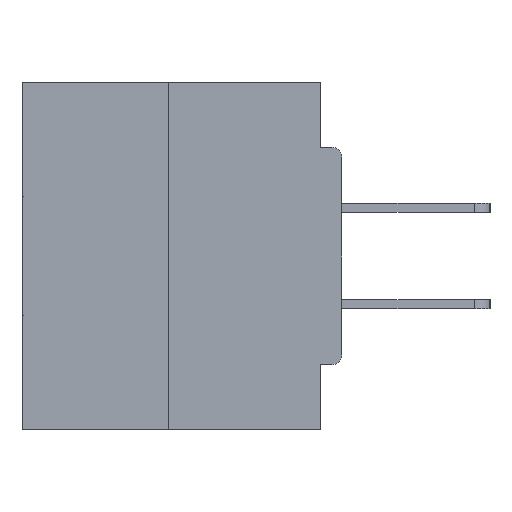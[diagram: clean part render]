
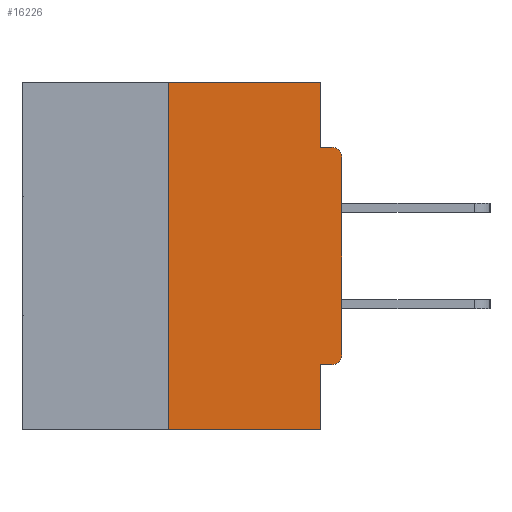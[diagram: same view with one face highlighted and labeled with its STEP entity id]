
A CAD part, left-side view. The second image highlights one B-rep face of the part: STEP entity #16226.
In plain terms, the highlighted planar face has unit normal (-1, 0, 0).
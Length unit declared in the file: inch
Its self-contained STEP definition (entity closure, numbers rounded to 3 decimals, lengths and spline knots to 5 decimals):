
#726 = CARTESIAN_POINT ( 'NONE',  ( 0., 0.015, -0.4065 ) ) ;
#1632 = CIRCLE ( 'NONE', #24550, 0.015 ) ;
#4187 = VERTEX_POINT ( 'NONE', #37827 ) ;
#4251 = EDGE_CURVE ( 'NONE', #29458, #31498, #21934, .T. ) ;
#4314 = EDGE_CURVE ( 'NONE', #35933, #25921, #5389, .T. ) ;
#4438 = LINE ( 'NONE', #27031, #31318 ) ;
#4513 = ORIENTED_EDGE ( 'NONE', *, *, #22392, .T. ) ;
#4729 = VERTEX_POINT ( 'NONE', #14237 ) ;
#4749 = DIRECTION ( 'NONE',  ( 0., 0., -1. ) ) ;
#5389 = LINE ( 'NONE', #38751, #9165 ) ;
#6288 = EDGE_CURVE ( 'NONE', #29458, #33371, #18903, .T. ) ;
#6418 = CARTESIAN_POINT ( 'NONE',  ( 0., 0., -0.3915 ) ) ;
#8263 = DIRECTION ( 'NONE',  ( 1., 0., 0. ) ) ;
#9165 = VECTOR ( 'NONE', #26657, 39.37008 ) ;
#9715 = VECTOR ( 'NONE', #4749, 39.37008 ) ;
#10452 = CARTESIAN_POINT ( 'NONE',  ( 0., 0.25, 0. ) ) ;
#10762 = FACE_OUTER_BOUND ( 'NONE', #16649, .T. ) ;
#10782 = CARTESIAN_POINT ( 'NONE',  ( 0., 0.015, -0.0935 ) ) ;
#11298 = DIRECTION ( 'NONE',  ( 0., -1., 0. ) ) ;
#11410 = CARTESIAN_POINT ( 'NONE',  ( 0., 0.015, -0.1085 ) ) ;
#11982 = DIRECTION ( 'NONE',  ( 0., -1., 0. ) ) ;
#13202 = VERTEX_POINT ( 'NONE', #36590 ) ;
#13882 = VECTOR ( 'NONE', #20357, 39.37008 ) ;
#14084 = LINE ( 'NONE', #37964, #38098 ) ;
#14098 = CARTESIAN_POINT ( 'NONE',  ( 0., 0.46, 0. ) ) ;
#14237 = CARTESIAN_POINT ( 'NONE',  ( 0., 0.031, -0.5 ) ) ;
#15349 = CARTESIAN_POINT ( 'NONE',  ( 0., 0.031, 0. ) ) ;
#16226 = ADVANCED_FACE ( 'NONE', ( #10762 ), #38574, .F. ) ;
#16649 = EDGE_LOOP ( 'NONE', ( #32845, #31484, #32725, #24927, #24960, #26338, #16756, #4513, #18245, #19762 ) ) ;
#16756 = ORIENTED_EDGE ( 'NONE', *, *, #21710, .T. ) ;
#16948 = CARTESIAN_POINT ( 'NONE',  ( 0., 0.25, 0. ) ) ;
#17215 = DIRECTION ( 'NONE',  ( 0., 0., -1. ) ) ;
#17398 = AXIS2_PLACEMENT_3D ( 'NONE', #31914, #35053, #37705 ) ;
#18002 = DIRECTION ( 'NONE',  ( 0., 0., 1. ) ) ;
#18245 = ORIENTED_EDGE ( 'NONE', *, *, #24643, .F. ) ;
#18903 = CIRCLE ( 'NONE', #17398, 0.015 ) ;
#19762 = ORIENTED_EDGE ( 'NONE', *, *, #34232, .F. ) ;
#20177 = DIRECTION ( 'NONE',  ( 0., 0., -1. ) ) ;
#20357 = DIRECTION ( 'NONE',  ( 0., 1., 0. ) ) ;
#20822 = CARTESIAN_POINT ( 'NONE',  ( 0., 0.031, -0.4065 ) ) ;
#21710 = EDGE_CURVE ( 'NONE', #33371, #13202, #27194, .T. ) ;
#21934 = LINE ( 'NONE', #26002, #13882 ) ;
#22392 = EDGE_CURVE ( 'NONE', #13202, #37519, #1632, .T. ) ;
#23120 = CARTESIAN_POINT ( 'NONE',  ( 0., 0.031, -0.5 ) ) ;
#23213 = LINE ( 'NONE', #26319, #30232 ) ;
#24550 = AXIS2_PLACEMENT_3D ( 'NONE', #11410, #35357, #17215 ) ;
#24643 = EDGE_CURVE ( 'NONE', #4187, #37519, #4438, .T. ) ;
#24927 = ORIENTED_EDGE ( 'NONE', *, *, #35275, .F. ) ;
#24960 = ORIENTED_EDGE ( 'NONE', *, *, #4251, .F. ) ;
#25842 = EDGE_CURVE ( 'NONE', #33291, #35933, #35011, .T. ) ;
#25921 = VERTEX_POINT ( 'NONE', #15349 ) ;
#26002 = CARTESIAN_POINT ( 'NONE',  ( 0., 0., -0.4065 ) ) ;
#26319 = CARTESIAN_POINT ( 'NONE',  ( 0., 0.46, -0.5 ) ) ;
#26338 = ORIENTED_EDGE ( 'NONE', *, *, #6288, .T. ) ;
#26657 = DIRECTION ( 'NONE',  ( 0., -1., 0. ) ) ;
#26762 = CARTESIAN_POINT ( 'NONE',  ( 0., 0.25, -0.5 ) ) ;
#27031 = CARTESIAN_POINT ( 'NONE',  ( 0., 0., -0.0935 ) ) ;
#27194 = LINE ( 'NONE', #37994, #35166 ) ;
#29331 = VECTOR ( 'NONE', #34945, 39.37008 ) ;
#29422 = AXIS2_PLACEMENT_3D ( 'NONE', #14098, #8263, #20177 ) ;
#29458 = VERTEX_POINT ( 'NONE', #726 ) ;
#30232 = VECTOR ( 'NONE', #11298, 39.37008 ) ;
#31318 = VECTOR ( 'NONE', #11982, 39.37008 ) ;
#31484 = ORIENTED_EDGE ( 'NONE', *, *, #25842, .F. ) ;
#31498 = VERTEX_POINT ( 'NONE', #20822 ) ;
#31914 = CARTESIAN_POINT ( 'NONE',  ( 0., 0.015, -0.3915 ) ) ;
#32269 = EDGE_CURVE ( 'NONE', #33291, #4729, #23213, .T. ) ;
#32725 = ORIENTED_EDGE ( 'NONE', *, *, #32269, .T. ) ;
#32845 = ORIENTED_EDGE ( 'NONE', *, *, #4314, .F. ) ;
#33291 = VERTEX_POINT ( 'NONE', #26762 ) ;
#33371 = VERTEX_POINT ( 'NONE', #6418 ) ;
#34232 = EDGE_CURVE ( 'NONE', #25921, #4187, #14084, .T. ) ;
#34945 = DIRECTION ( 'NONE',  ( 0., 0., 1. ) ) ;
#35011 = LINE ( 'NONE', #16948, #29331 ) ;
#35053 = DIRECTION ( 'NONE',  ( -1., 0., 0. ) ) ;
#35166 = VECTOR ( 'NONE', #18002, 39.37008 ) ;
#35195 = DIRECTION ( 'NONE',  ( 0., 0., -1. ) ) ;
#35275 = EDGE_CURVE ( 'NONE', #31498, #4729, #36584, .T. ) ;
#35357 = DIRECTION ( 'NONE',  ( -1., 0., 0. ) ) ;
#35933 = VERTEX_POINT ( 'NONE', #10452 ) ;
#36584 = LINE ( 'NONE', #23120, #9715 ) ;
#36590 = CARTESIAN_POINT ( 'NONE',  ( 0., 0., -0.1085 ) ) ;
#37519 = VERTEX_POINT ( 'NONE', #10782 ) ;
#37705 = DIRECTION ( 'NONE',  ( 0., 0., -1. ) ) ;
#37827 = CARTESIAN_POINT ( 'NONE',  ( 0., 0.031, -0.0935 ) ) ;
#37964 = CARTESIAN_POINT ( 'NONE',  ( 0., 0.031, 0. ) ) ;
#37994 = CARTESIAN_POINT ( 'NONE',  ( 0., 0., 0. ) ) ;
#38098 = VECTOR ( 'NONE', #35195, 39.37008 ) ;
#38574 = PLANE ( 'NONE',  #29422 ) ;
#38751 = CARTESIAN_POINT ( 'NONE',  ( 0., 0.46, 0. ) ) ;
